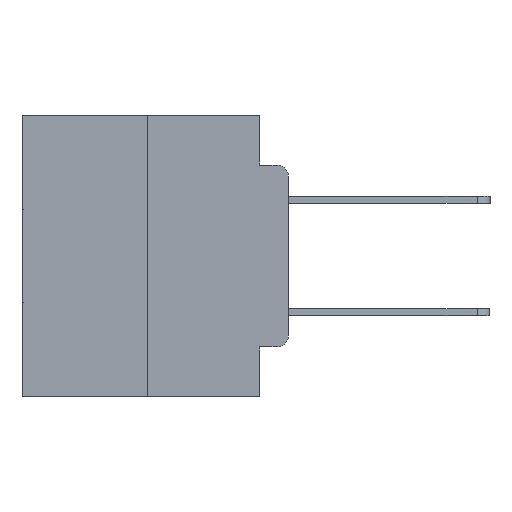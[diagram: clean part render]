
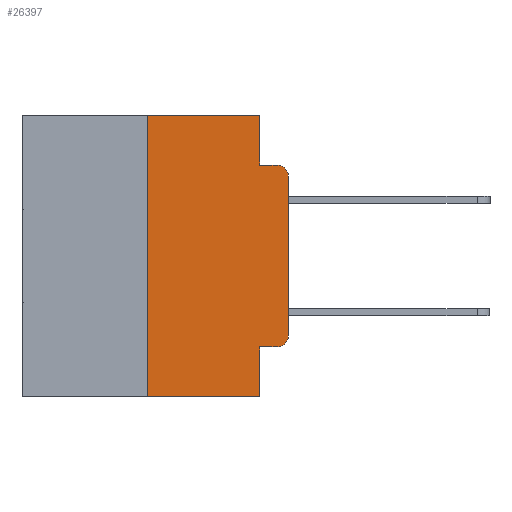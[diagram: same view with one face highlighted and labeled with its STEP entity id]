
A CAD part, left-side view. The second image highlights one B-rep face of the part: STEP entity #26397.
In plain terms, the highlighted planar face has unit normal (-1, 0, 0).
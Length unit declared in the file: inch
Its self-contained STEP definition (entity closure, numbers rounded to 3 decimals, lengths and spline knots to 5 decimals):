
#320 = ORIENTED_EDGE ( 'NONE', *, *, #28106, .T. ) ;
#672 = ORIENTED_EDGE ( 'NONE', *, *, #7725, .F. ) ;
#1038 = DIRECTION ( 'NONE',  ( 0., 0., -1. ) ) ;
#1457 = EDGE_CURVE ( 'NONE', #16659, #2957, #19460, .T. ) ;
#2300 = VECTOR ( 'NONE', #10191, 39.37008 ) ;
#2957 = VERTEX_POINT ( 'NONE', #11037 ) ;
#3041 = EDGE_CURVE ( 'NONE', #27273, #16704, #10370, .T. ) ;
#4482 = AXIS2_PLACEMENT_3D ( 'NONE', #13285, #6391, #22481 ) ;
#4619 = EDGE_CURVE ( 'NONE', #27035, #5970, #16349, .T. ) ;
#5119 = ORIENTED_EDGE ( 'NONE', *, *, #1457, .F. ) ;
#5229 = DIRECTION ( 'NONE',  ( 0., 0., -1. ) ) ;
#5775 = CARTESIAN_POINT ( 'NONE',  ( 0., 0.051, -0.0885 ) ) ;
#5970 = VERTEX_POINT ( 'NONE', #5775 ) ;
#6391 = DIRECTION ( 'NONE',  ( 1., 0., 0. ) ) ;
#7725 = EDGE_CURVE ( 'NONE', #5970, #21750, #13320, .T. ) ;
#8033 = LINE ( 'NONE', #21926, #13457 ) ;
#8212 = VECTOR ( 'NONE', #27214, 39.37008 ) ;
#8917 = CARTESIAN_POINT ( 'NONE',  ( 0., 0.051, 0. ) ) ;
#9270 = EDGE_CURVE ( 'NONE', #10972, #21750, #27725, .T. ) ;
#9528 = DIRECTION ( 'NONE',  ( -1., 0., 0. ) ) ;
#9821 = ORIENTED_EDGE ( 'NONE', *, *, #3041, .F. ) ;
#10086 = EDGE_CURVE ( 'NONE', #27273, #2957, #10277, .T. ) ;
#10191 = DIRECTION ( 'NONE',  ( 0., -1., 0. ) ) ;
#10209 = DIRECTION ( 'NONE',  ( -1., 0., 0. ) ) ;
#10277 = LINE ( 'NONE', #24442, #23171 ) ;
#10370 = LINE ( 'NONE', #27118, #8212 ) ;
#10710 = CARTESIAN_POINT ( 'NONE',  ( 0., 0., -0.3915 ) ) ;
#10758 = DIRECTION ( 'NONE',  ( 0., -1., 0. ) ) ;
#10819 = EDGE_CURVE ( 'NONE', #27723, #10972, #21292, .T. ) ;
#10972 = VERTEX_POINT ( 'NONE', #23400 ) ;
#11037 = CARTESIAN_POINT ( 'NONE',  ( 0., 0.051, -0.5 ) ) ;
#11381 = DIRECTION ( 'NONE',  ( 0., 0., 1. ) ) ;
#11574 = DIRECTION ( 'NONE',  ( 0., -1., 0. ) ) ;
#11597 = ORIENTED_EDGE ( 'NONE', *, *, #10819, .T. ) ;
#12212 = CARTESIAN_POINT ( 'NONE',  ( 0., 0.051, 0. ) ) ;
#13035 = CARTESIAN_POINT ( 'NONE',  ( 0., 0.02, -0.4115 ) ) ;
#13285 = CARTESIAN_POINT ( 'NONE',  ( 0., 0.473, 0. ) ) ;
#13320 = LINE ( 'NONE', #25235, #24019 ) ;
#13364 = VECTOR ( 'NONE', #1038, 39.37008 ) ;
#13457 = VECTOR ( 'NONE', #15184, 39.37008 ) ;
#14868 = CARTESIAN_POINT ( 'NONE',  ( 0., 0.051, -0.4115 ) ) ;
#15184 = DIRECTION ( 'NONE',  ( 0., -1., 0. ) ) ;
#15426 = CARTESIAN_POINT ( 'NONE',  ( 0., 0.02, -0.0885 ) ) ;
#15748 = CARTESIAN_POINT ( 'NONE',  ( 0., 0.25, 0. ) ) ;
#15956 = VERTEX_POINT ( 'NONE', #13035 ) ;
#16349 = LINE ( 'NONE', #12212, #17065 ) ;
#16508 = EDGE_CURVE ( 'NONE', #16704, #27035, #8033, .T. ) ;
#16659 = VERTEX_POINT ( 'NONE', #24743 ) ;
#16704 = VERTEX_POINT ( 'NONE', #15748 ) ;
#17065 = VECTOR ( 'NONE', #5229, 39.37008 ) ;
#17276 = CARTESIAN_POINT ( 'NONE',  ( 0., 0.051, 0. ) ) ;
#18467 = ORIENTED_EDGE ( 'NONE', *, *, #9270, .T. ) ;
#19460 = LINE ( 'NONE', #17276, #13364 ) ;
#19897 = ORIENTED_EDGE ( 'NONE', *, *, #4619, .F. ) ;
#20132 = FACE_OUTER_BOUND ( 'NONE', #22662, .T. ) ;
#20598 = ORIENTED_EDGE ( 'NONE', *, *, #16508, .F. ) ;
#21292 = LINE ( 'NONE', #25040, #26549 ) ;
#21750 = VERTEX_POINT ( 'NONE', #15426 ) ;
#21926 = CARTESIAN_POINT ( 'NONE',  ( 0., 0.473, 0. ) ) ;
#22035 = ORIENTED_EDGE ( 'NONE', *, *, #10086, .T. ) ;
#22388 = PLANE ( 'NONE',  #4482 ) ;
#22481 = DIRECTION ( 'NONE',  ( 0., 0., -1. ) ) ;
#22662 = EDGE_LOOP ( 'NONE', ( #11597, #18467, #672, #19897, #20598, #9821, #22035, #5119, #320, #24827 ) ) ;
#22960 = AXIS2_PLACEMENT_3D ( 'NONE', #23242, #9528, #25471 ) ;
#23171 = VECTOR ( 'NONE', #10758, 39.37008 ) ;
#23242 = CARTESIAN_POINT ( 'NONE',  ( 0., 0.02, -0.3915 ) ) ;
#23400 = CARTESIAN_POINT ( 'NONE',  ( 0., 0., -0.1085 ) ) ;
#23463 = AXIS2_PLACEMENT_3D ( 'NONE', #23912, #10209, #26143 ) ;
#23912 = CARTESIAN_POINT ( 'NONE',  ( 0., 0.02, -0.1085 ) ) ;
#24019 = VECTOR ( 'NONE', #11574, 39.37008 ) ;
#24442 = CARTESIAN_POINT ( 'NONE',  ( 0., 0.473, -0.5 ) ) ;
#24743 = CARTESIAN_POINT ( 'NONE',  ( 0., 0.051, -0.4115 ) ) ;
#24827 = ORIENTED_EDGE ( 'NONE', *, *, #26635, .T. ) ;
#25040 = CARTESIAN_POINT ( 'NONE',  ( 0., 0., 0. ) ) ;
#25235 = CARTESIAN_POINT ( 'NONE',  ( 0., 0.051, -0.0885 ) ) ;
#25471 = DIRECTION ( 'NONE',  ( 0., 0., -1. ) ) ;
#25729 = CARTESIAN_POINT ( 'NONE',  ( 0., 0.25, -0.5 ) ) ;
#25733 = CIRCLE ( 'NONE', #22960, 0.02 ) ;
#25986 = LINE ( 'NONE', #14868, #2300 ) ;
#26143 = DIRECTION ( 'NONE',  ( 0., 0., -1. ) ) ;
#26397 = ADVANCED_FACE ( 'NONE', ( #20132 ), #22388, .F. ) ;
#26549 = VECTOR ( 'NONE', #11381, 39.37008 ) ;
#26635 = EDGE_CURVE ( 'NONE', #15956, #27723, #25733, .T. ) ;
#27035 = VERTEX_POINT ( 'NONE', #8917 ) ;
#27118 = CARTESIAN_POINT ( 'NONE',  ( 0., 0.25, 0. ) ) ;
#27214 = DIRECTION ( 'NONE',  ( 0., 0., 1. ) ) ;
#27273 = VERTEX_POINT ( 'NONE', #25729 ) ;
#27723 = VERTEX_POINT ( 'NONE', #10710 ) ;
#27725 = CIRCLE ( 'NONE', #23463, 0.02 ) ;
#28106 = EDGE_CURVE ( 'NONE', #16659, #15956, #25986, .T. ) ;
